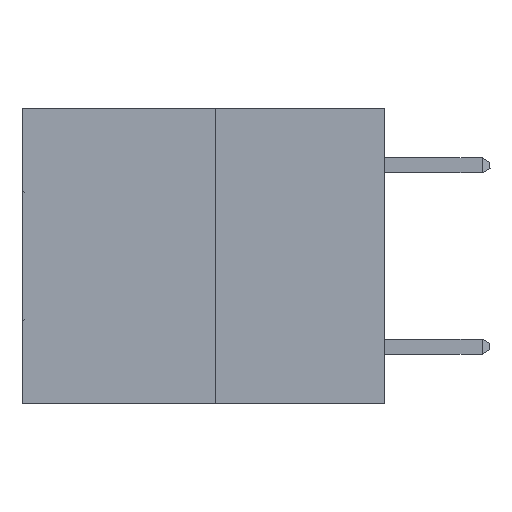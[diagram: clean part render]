
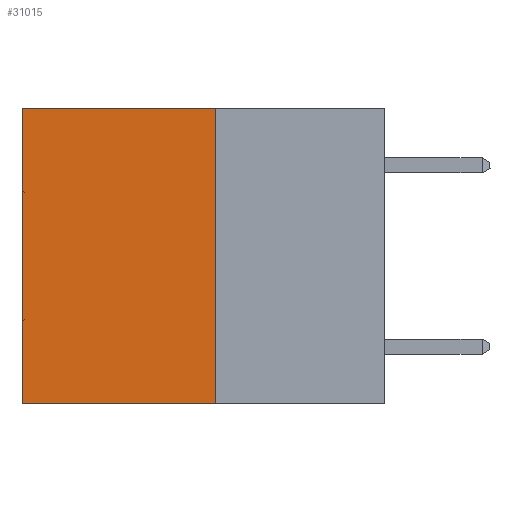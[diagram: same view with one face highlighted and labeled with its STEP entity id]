
A CAD part, left-side view. The second image highlights one B-rep face of the part: STEP entity #31015.
In plain terms, the highlighted planar face has unit normal (-1, 0, 0).
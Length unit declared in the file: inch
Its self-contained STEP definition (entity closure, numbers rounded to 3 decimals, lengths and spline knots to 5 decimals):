
#585 = AXIS2_PLACEMENT_3D ( 'NONE', #29346, #13272, #15797 ) ;
#756 = LINE ( 'NONE', #18232, #13009 ) ;
#6123 = VERTEX_POINT ( 'NONE', #7025 ) ;
#6696 = ORIENTED_EDGE ( 'NONE', *, *, #17716, .F. ) ;
#7025 = CARTESIAN_POINT ( 'NONE',  ( 0.3165, 0.28, -0.49 ) ) ;
#8223 = PLANE ( 'NONE',  #585 ) ;
#8444 = VERTEX_POINT ( 'NONE', #17087 ) ;
#8719 = VECTOR ( 'NONE', #22371, 39.37008 ) ;
#10095 = DIRECTION ( 'NONE',  ( 0., 1., 0. ) ) ;
#11191 = VECTOR ( 'NONE', #17157, 39.37008 ) ;
#13009 = VECTOR ( 'NONE', #15214, 39.37008 ) ;
#13154 = EDGE_CURVE ( 'NONE', #21163, #8444, #28972, .T. ) ;
#13212 = EDGE_CURVE ( 'NONE', #21163, #6123, #31513, .T. ) ;
#13272 = DIRECTION ( 'NONE',  ( 1., 0., 0. ) ) ;
#15214 = DIRECTION ( 'NONE',  ( 0., 0., -1. ) ) ;
#15797 = DIRECTION ( 'NONE',  ( 0., 0., -1. ) ) ;
#16991 = EDGE_LOOP ( 'NONE', ( #20086, #6696, #17261, #30886 ) ) ;
#17087 = CARTESIAN_POINT ( 'NONE',  ( 0.3165, 0.6, 0. ) ) ;
#17157 = DIRECTION ( 'NONE',  ( 0., 0., -1. ) ) ;
#17261 = ORIENTED_EDGE ( 'NONE', *, *, #13212, .F. ) ;
#17324 = VECTOR ( 'NONE', #10095, 39.37008 ) ;
#17716 = EDGE_CURVE ( 'NONE', #6123, #24162, #19021, .T. ) ;
#18232 = CARTESIAN_POINT ( 'NONE',  ( 0.3165, 0.6, -0.49 ) ) ;
#19021 = LINE ( 'NONE', #24176, #17324 ) ;
#19742 = CARTESIAN_POINT ( 'NONE',  ( 0.3165, 0.28, -0.49 ) ) ;
#20086 = ORIENTED_EDGE ( 'NONE', *, *, #31821, .T. ) ;
#21163 = VERTEX_POINT ( 'NONE', #29516 ) ;
#22371 = DIRECTION ( 'NONE',  ( 0., 1., 0. ) ) ;
#24162 = VERTEX_POINT ( 'NONE', #34119 ) ;
#24176 = CARTESIAN_POINT ( 'NONE',  ( 0.3165, 0.28, -0.49 ) ) ;
#28972 = LINE ( 'NONE', #33336, #8719 ) ;
#29346 = CARTESIAN_POINT ( 'NONE',  ( 0.3165, 0.28, -0.49 ) ) ;
#29516 = CARTESIAN_POINT ( 'NONE',  ( 0.3165, 0.28, 0. ) ) ;
#30527 = FACE_OUTER_BOUND ( 'NONE', #16991, .T. ) ;
#30886 = ORIENTED_EDGE ( 'NONE', *, *, #13154, .T. ) ;
#31015 = ADVANCED_FACE ( 'NONE', ( #30527 ), #8223, .F. ) ;
#31513 = LINE ( 'NONE', #19742, #11191 ) ;
#31821 = EDGE_CURVE ( 'NONE', #8444, #24162, #756, .T. ) ;
#33336 = CARTESIAN_POINT ( 'NONE',  ( 0.3165, 0.28, 0. ) ) ;
#34119 = CARTESIAN_POINT ( 'NONE',  ( 0.3165, 0.6, -0.49 ) ) ;
